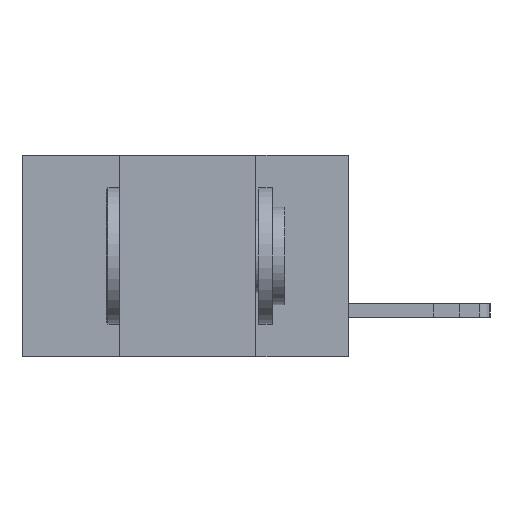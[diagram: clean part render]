
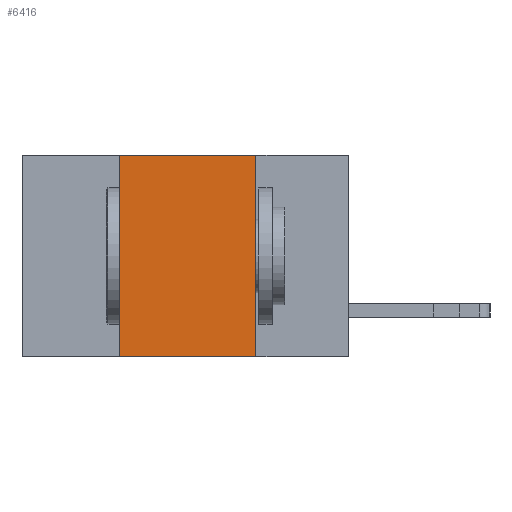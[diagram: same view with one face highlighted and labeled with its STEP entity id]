
A CAD part, left-side view. The second image highlights one B-rep face of the part: STEP entity #6416.
In plain terms, the highlighted planar face has unit normal (-1, 0, 0).
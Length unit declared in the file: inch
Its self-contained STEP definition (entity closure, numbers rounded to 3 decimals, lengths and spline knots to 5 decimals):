
#589 = CARTESIAN_POINT ( 'NONE',  ( 0., 0.17, 0. ) ) ;
#732 = FACE_OUTER_BOUND ( 'NONE', #5789, .T. ) ;
#1814 = ORIENTED_EDGE ( 'NONE', *, *, #8336, .F. ) ;
#2190 = DIRECTION ( 'NONE',  ( 0., 0., 1. ) ) ;
#2580 = CARTESIAN_POINT ( 'NONE',  ( 0., 0.6, -0.37 ) ) ;
#2698 = CARTESIAN_POINT ( 'NONE',  ( 0., 0.42, 0. ) ) ;
#2728 = VERTEX_POINT ( 'NONE', #2774 ) ;
#2774 = CARTESIAN_POINT ( 'NONE',  ( 0., 0.42, -0.37 ) ) ;
#2860 = ORIENTED_EDGE ( 'NONE', *, *, #9733, .T. ) ;
#2980 = CARTESIAN_POINT ( 'NONE',  ( 0., 0.6, 0. ) ) ;
#3711 = VECTOR ( 'NONE', #10863, 39.37008 ) ;
#3830 = LINE ( 'NONE', #589, #10742 ) ;
#3915 = CARTESIAN_POINT ( 'NONE',  ( 0., 0.42, 0. ) ) ;
#3917 = VERTEX_POINT ( 'NONE', #6038 ) ;
#4052 = EDGE_CURVE ( 'NONE', #2728, #4688, #9293, .T. ) ;
#4112 = ORIENTED_EDGE ( 'NONE', *, *, #4052, .F. ) ;
#4688 = VERTEX_POINT ( 'NONE', #3915 ) ;
#5061 = PLANE ( 'NONE',  #5548 ) ;
#5162 = DIRECTION ( 'NONE',  ( 0., 0., -1. ) ) ;
#5207 = EDGE_CURVE ( 'NONE', #4688, #10469, #6434, .T. ) ;
#5548 = AXIS2_PLACEMENT_3D ( 'NONE', #2980, #6440, #7876 ) ;
#5653 = CARTESIAN_POINT ( 'NONE',  ( 0., 0.17, 0. ) ) ;
#5789 = EDGE_LOOP ( 'NONE', ( #1814, #10587, #4112, #2860 ) ) ;
#6038 = CARTESIAN_POINT ( 'NONE',  ( 0., 0.17, -0.37 ) ) ;
#6416 = ADVANCED_FACE ( 'NONE', ( #732 ), #5061, .F. ) ;
#6434 = LINE ( 'NONE', #11037, #3711 ) ;
#6440 = DIRECTION ( 'NONE',  ( 1., 0., 0. ) ) ;
#7876 = DIRECTION ( 'NONE',  ( 0., 0., -1. ) ) ;
#8336 = EDGE_CURVE ( 'NONE', #10469, #3917, #3830, .T. ) ;
#9293 = LINE ( 'NONE', #2698, #11319 ) ;
#9343 = VECTOR ( 'NONE', #11573, 39.37008 ) ;
#9733 = EDGE_CURVE ( 'NONE', #2728, #3917, #11623, .T. ) ;
#10469 = VERTEX_POINT ( 'NONE', #5653 ) ;
#10587 = ORIENTED_EDGE ( 'NONE', *, *, #5207, .F. ) ;
#10742 = VECTOR ( 'NONE', #5162, 39.37008 ) ;
#10863 = DIRECTION ( 'NONE',  ( 0., -1., 0. ) ) ;
#11037 = CARTESIAN_POINT ( 'NONE',  ( 0., 0.6, 0. ) ) ;
#11319 = VECTOR ( 'NONE', #2190, 39.37008 ) ;
#11573 = DIRECTION ( 'NONE',  ( 0., -1., 0. ) ) ;
#11623 = LINE ( 'NONE', #2580, #9343 ) ;
